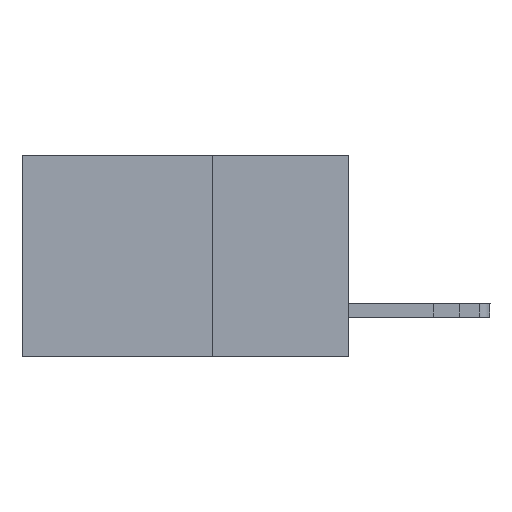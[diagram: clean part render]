
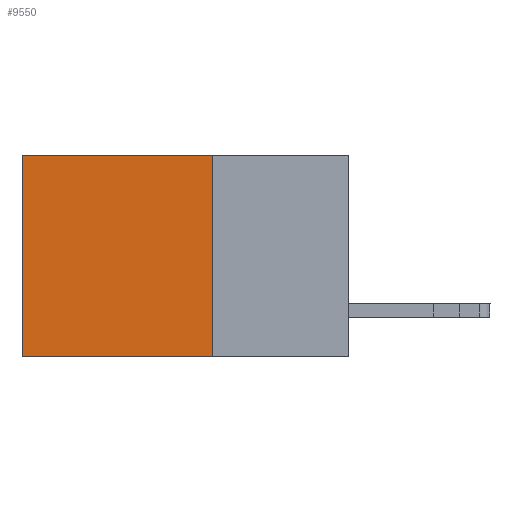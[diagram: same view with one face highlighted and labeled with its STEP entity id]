
A CAD part, left-side view. The second image highlights one B-rep face of the part: STEP entity #9550.
In plain terms, the highlighted planar face has unit normal (-1, 0, 0).
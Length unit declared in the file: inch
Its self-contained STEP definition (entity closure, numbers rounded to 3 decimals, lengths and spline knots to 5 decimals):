
#1149 = VERTEX_POINT ( 'NONE', #6326 ) ;
#1476 = CARTESIAN_POINT ( 'NONE',  ( 0.2615, 0.25, 0. ) ) ;
#1569 = DIRECTION ( 'NONE',  ( 0., 0., -1. ) ) ;
#1747 = VERTEX_POINT ( 'NONE', #7535 ) ;
#2307 = AXIS2_PLACEMENT_3D ( 'NONE', #17385, #10068, #1569 ) ;
#2622 = ORIENTED_EDGE ( 'NONE', *, *, #14717, .T. ) ;
#3180 = LINE ( 'NONE', #15155, #13824 ) ;
#4628 = LINE ( 'NONE', #13379, #11529 ) ;
#5333 = EDGE_CURVE ( 'NONE', #1747, #1149, #15536, .T. ) ;
#6326 = CARTESIAN_POINT ( 'NONE',  ( 0.2615, 0.6, -0.37 ) ) ;
#6486 = EDGE_LOOP ( 'NONE', ( #11097, #16643, #8953, #2622 ) ) ;
#6521 = DIRECTION ( 'NONE',  ( 0., 0., -1. ) ) ;
#7379 = VECTOR ( 'NONE', #14957, 39.37008 ) ;
#7535 = CARTESIAN_POINT ( 'NONE',  ( 0.2615, 0.25, -0.37 ) ) ;
#8206 = EDGE_CURVE ( 'NONE', #13727, #1747, #3180, .T. ) ;
#8297 = VECTOR ( 'NONE', #10502, 39.37008 ) ;
#8953 = ORIENTED_EDGE ( 'NONE', *, *, #8206, .F. ) ;
#9550 = ADVANCED_FACE ( 'NONE', ( #13150 ), #14079, .F. ) ;
#9680 = DIRECTION ( 'NONE',  ( 0., 0., -1. ) ) ;
#10068 = DIRECTION ( 'NONE',  ( 1., 0., 0. ) ) ;
#10502 = DIRECTION ( 'NONE',  ( 0., 1., 0. ) ) ;
#11015 = LINE ( 'NONE', #13597, #7379 ) ;
#11097 = ORIENTED_EDGE ( 'NONE', *, *, #12083, .T. ) ;
#11114 = VERTEX_POINT ( 'NONE', #14961 ) ;
#11529 = VECTOR ( 'NONE', #6521, 39.37008 ) ;
#12083 = EDGE_CURVE ( 'NONE', #11114, #1149, #4628, .T. ) ;
#13150 = FACE_OUTER_BOUND ( 'NONE', #6486, .T. ) ;
#13379 = CARTESIAN_POINT ( 'NONE',  ( 0.2615, 0.6, -0.37 ) ) ;
#13597 = CARTESIAN_POINT ( 'NONE',  ( 0.2615, 0.25, 0. ) ) ;
#13727 = VERTEX_POINT ( 'NONE', #1476 ) ;
#13824 = VECTOR ( 'NONE', #9680, 39.37008 ) ;
#14079 = PLANE ( 'NONE',  #2307 ) ;
#14717 = EDGE_CURVE ( 'NONE', #13727, #11114, #11015, .T. ) ;
#14957 = DIRECTION ( 'NONE',  ( 0., 1., 0. ) ) ;
#14961 = CARTESIAN_POINT ( 'NONE',  ( 0.2615, 0.6, 0. ) ) ;
#15155 = CARTESIAN_POINT ( 'NONE',  ( 0.2615, 0.25, -0.37 ) ) ;
#15536 = LINE ( 'NONE', #17221, #8297 ) ;
#16643 = ORIENTED_EDGE ( 'NONE', *, *, #5333, .F. ) ;
#17221 = CARTESIAN_POINT ( 'NONE',  ( 0.2615, 0.25, -0.37 ) ) ;
#17385 = CARTESIAN_POINT ( 'NONE',  ( 0.2615, 0.25, -0.37 ) ) ;
